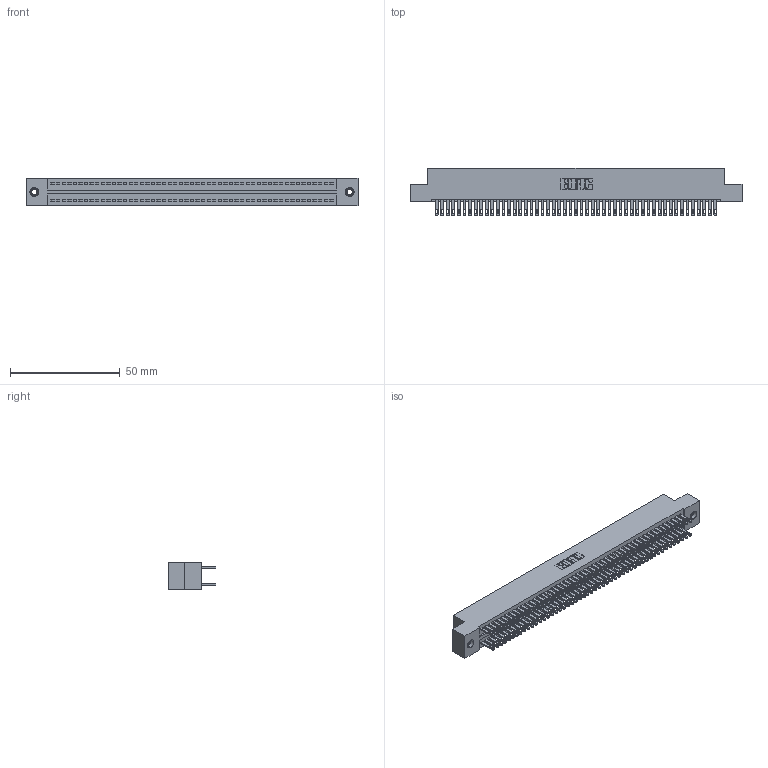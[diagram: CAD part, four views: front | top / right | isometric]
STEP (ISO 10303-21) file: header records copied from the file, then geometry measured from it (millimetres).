
FILE_DESCRIPTION (( 'STEP AP203' ), '1' );
FILE_NAME ('325-102-500-207.STEP', '2020-02-25T06:45:45', ( '' ), ( '' ), 'SwSTEP 2.0', 'SolidWorks 2016', '' );
FILE_SCHEMA (( 'CONFIG_CONTROL_DESIGN' ));
Length unit declared in the file: inch
Products named in the file (4): 325 Part_TI; 325-102-500-207; 345-250-001_345-250-005-103; 325-292-001_325-293-100
Assembly tree (105 placements, depth 2):
  325-102-500-207
    325 Part_TI
    325-292-001_325-293-100  x102
    345-250-001_345-250-005-103  x2
Bounding box: 151.26 x 21.84 x 12.45 mm (x, y, z)
Volume: 19905.6 mm3; surface area: 25399.2 mm2
Topology: 105 solids, 105 shells, 5070 faces, 15441 edges, 10286 vertices
Faces by surface type: plane 3162, cylinder 1892, cone 12, torus 4
Entity records: 32762 total; most frequent: CARTESIAN_POINT 5401, ORIENTED_EDGE 5330, DIRECTION 4631, EDGE_CURVE 2665, LINE 2513, VECTOR 2513, VERTEX_POINT 1772, AXIS2_PLACEMENT_3D 1059
